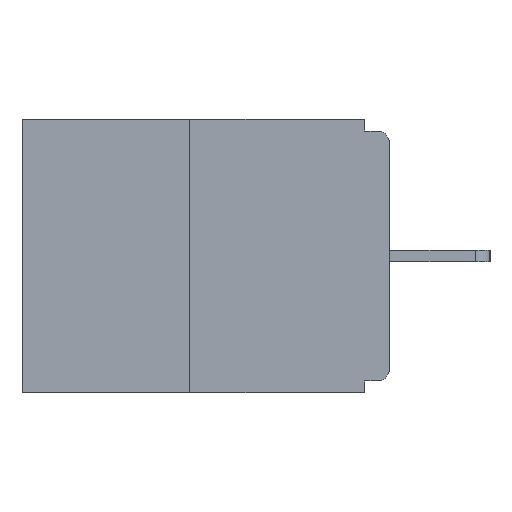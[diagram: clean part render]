
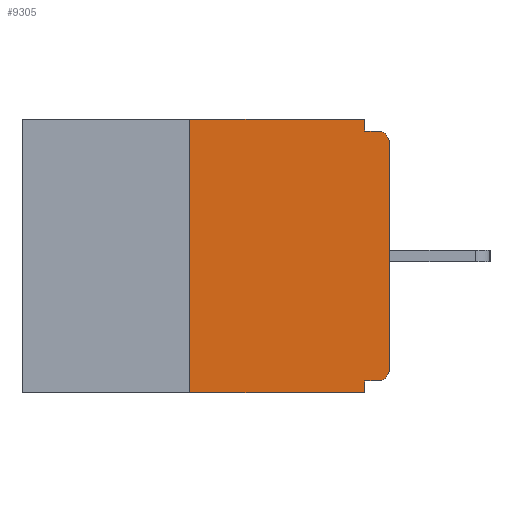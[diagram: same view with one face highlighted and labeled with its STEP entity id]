
A CAD part, left-side view. The second image highlights one B-rep face of the part: STEP entity #9305.
In plain terms, the highlighted planar face has unit normal (-1, 0, 0).
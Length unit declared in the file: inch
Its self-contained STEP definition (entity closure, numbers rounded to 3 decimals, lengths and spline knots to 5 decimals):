
#163 = DIRECTION ( 'NONE',  ( 0., -1., 0. ) ) ;
#285 = VERTEX_POINT ( 'NONE', #2103 ) ;
#522 = EDGE_CURVE ( 'NONE', #285, #22776, #17040, .T. ) ;
#612 = DIRECTION ( 'NONE',  ( 0., 0., -1. ) ) ;
#1006 = CARTESIAN_POINT ( 'NONE',  ( 0., 0.25, 0. ) ) ;
#1192 = LINE ( 'NONE', #10420, #7097 ) ;
#1341 = DIRECTION ( 'NONE',  ( 0., 1., 0. ) ) ;
#1607 = VERTEX_POINT ( 'NONE', #23105 ) ;
#1938 = DIRECTION ( 'NONE',  ( -1., 0., 0. ) ) ;
#2103 = CARTESIAN_POINT ( 'NONE',  ( 0., 0.25, -0.343 ) ) ;
#2117 = ORIENTED_EDGE ( 'NONE', *, *, #6158, .F. ) ;
#3334 = VECTOR ( 'NONE', #4882, 39.37008 ) ;
#4086 = CARTESIAN_POINT ( 'NONE',  ( 0., 0.46, 0. ) ) ;
#4260 = CARTESIAN_POINT ( 'NONE',  ( 0., 0.031, -0.328 ) ) ;
#4323 = DIRECTION ( 'NONE',  ( -1., 0., 0. ) ) ;
#4334 = PLANE ( 'NONE',  #9970 ) ;
#4555 = VERTEX_POINT ( 'NONE', #4260 ) ;
#4598 = AXIS2_PLACEMENT_3D ( 'NONE', #17822, #4323, #9831 ) ;
#4882 = DIRECTION ( 'NONE',  ( 0., 0., -1. ) ) ;
#5003 = LINE ( 'NONE', #12257, #3334 ) ;
#5494 = VERTEX_POINT ( 'NONE', #14697 ) ;
#5523 = ORIENTED_EDGE ( 'NONE', *, *, #24624, .T. ) ;
#5715 = ORIENTED_EDGE ( 'NONE', *, *, #16537, .T. ) ;
#6006 = CARTESIAN_POINT ( 'NONE',  ( 0., 0., -0.03 ) ) ;
#6082 = DIRECTION ( 'NONE',  ( 1., 0., 0. ) ) ;
#6158 = EDGE_CURVE ( 'NONE', #17249, #1607, #17245, .T. ) ;
#6559 = ORIENTED_EDGE ( 'NONE', *, *, #17061, .F. ) ;
#6820 = LINE ( 'NONE', #8567, #7460 ) ;
#7097 = VECTOR ( 'NONE', #8794, 39.37008 ) ;
#7415 = EDGE_CURVE ( 'NONE', #22776, #17249, #22381, .T. ) ;
#7460 = VECTOR ( 'NONE', #1341, 39.37008 ) ;
#7556 = CARTESIAN_POINT ( 'NONE',  ( 0., 0.015, -0.03 ) ) ;
#7636 = ORIENTED_EDGE ( 'NONE', *, *, #7415, .F. ) ;
#8252 = EDGE_CURVE ( 'NONE', #1607, #5494, #13034, .T. ) ;
#8452 = VERTEX_POINT ( 'NONE', #11905 ) ;
#8567 = CARTESIAN_POINT ( 'NONE',  ( 0., 0., -0.328 ) ) ;
#8794 = DIRECTION ( 'NONE',  ( 0., -1., 0. ) ) ;
#8797 = CARTESIAN_POINT ( 'NONE',  ( 0., 0., -0.313 ) ) ;
#9305 = ADVANCED_FACE ( 'NONE', ( #10086 ), #4334, .F. ) ;
#9831 = DIRECTION ( 'NONE',  ( 0., 0., -1. ) ) ;
#9891 = DIRECTION ( 'NONE',  ( 0., 0., -1. ) ) ;
#9970 = AXIS2_PLACEMENT_3D ( 'NONE', #4086, #6082, #612 ) ;
#10086 = FACE_OUTER_BOUND ( 'NONE', #13972, .T. ) ;
#10420 = CARTESIAN_POINT ( 'NONE',  ( 0., 0.46, -0.343 ) ) ;
#11234 = ORIENTED_EDGE ( 'NONE', *, *, #16095, .F. ) ;
#11454 = DIRECTION ( 'NONE',  ( 0., 0., 1. ) ) ;
#11485 = ORIENTED_EDGE ( 'NONE', *, *, #522, .F. ) ;
#11905 = CARTESIAN_POINT ( 'NONE',  ( 0., 0.015, -0.328 ) ) ;
#11989 = CARTESIAN_POINT ( 'NONE',  ( 0., 0.031, -0.343 ) ) ;
#12257 = CARTESIAN_POINT ( 'NONE',  ( 0., 0.031, -0.343 ) ) ;
#12744 = ORIENTED_EDGE ( 'NONE', *, *, #19998, .T. ) ;
#13034 = LINE ( 'NONE', #17250, #19500 ) ;
#13067 = DIRECTION ( 'NONE',  ( 0., 0., 1. ) ) ;
#13758 = CARTESIAN_POINT ( 'NONE',  ( 0., 0.031, 0. ) ) ;
#13887 = ORIENTED_EDGE ( 'NONE', *, *, #8252, .F. ) ;
#13972 = EDGE_LOOP ( 'NONE', ( #7636, #11485, #5715, #6559, #11234, #21787, #12744, #5523, #13887, #2117 ) ) ;
#14697 = CARTESIAN_POINT ( 'NONE',  ( 0., 0.015, -0.015 ) ) ;
#15060 = CARTESIAN_POINT ( 'NONE',  ( 0., 0., 0. ) ) ;
#15184 = LINE ( 'NONE', #15060, #22370 ) ;
#15350 = CIRCLE ( 'NONE', #4598, 0.015 ) ;
#16095 = EDGE_CURVE ( 'NONE', #8452, #4555, #6820, .T. ) ;
#16537 = EDGE_CURVE ( 'NONE', #285, #24034, #1192, .T. ) ;
#16689 = CARTESIAN_POINT ( 'NONE',  ( 0., 0.25, 0. ) ) ;
#17040 = LINE ( 'NONE', #16689, #21193 ) ;
#17061 = EDGE_CURVE ( 'NONE', #4555, #24034, #5003, .T. ) ;
#17245 = LINE ( 'NONE', #13758, #23815 ) ;
#17249 = VERTEX_POINT ( 'NONE', #21214 ) ;
#17250 = CARTESIAN_POINT ( 'NONE',  ( 0., 0., -0.015 ) ) ;
#17822 = CARTESIAN_POINT ( 'NONE',  ( 0., 0.015, -0.313 ) ) ;
#17848 = VERTEX_POINT ( 'NONE', #8797 ) ;
#18068 = VERTEX_POINT ( 'NONE', #6006 ) ;
#18282 = VECTOR ( 'NONE', #20985, 39.37008 ) ;
#19500 = VECTOR ( 'NONE', #163, 39.37008 ) ;
#19998 = EDGE_CURVE ( 'NONE', #17848, #18068, #15184, .T. ) ;
#20985 = DIRECTION ( 'NONE',  ( 0., -1., 0. ) ) ;
#21193 = VECTOR ( 'NONE', #13067, 39.37008 ) ;
#21214 = CARTESIAN_POINT ( 'NONE',  ( 0., 0.031, 0. ) ) ;
#21292 = AXIS2_PLACEMENT_3D ( 'NONE', #7556, #1938, #24303 ) ;
#21787 = ORIENTED_EDGE ( 'NONE', *, *, #24415, .T. ) ;
#22370 = VECTOR ( 'NONE', #11454, 39.37008 ) ;
#22381 = LINE ( 'NONE', #22613, #18282 ) ;
#22613 = CARTESIAN_POINT ( 'NONE',  ( 0., 0.46, 0. ) ) ;
#22776 = VERTEX_POINT ( 'NONE', #1006 ) ;
#23105 = CARTESIAN_POINT ( 'NONE',  ( 0., 0.031, -0.015 ) ) ;
#23815 = VECTOR ( 'NONE', #9891, 39.37008 ) ;
#24034 = VERTEX_POINT ( 'NONE', #11989 ) ;
#24303 = DIRECTION ( 'NONE',  ( 0., 0., -1. ) ) ;
#24415 = EDGE_CURVE ( 'NONE', #8452, #17848, #15350, .T. ) ;
#24479 = CIRCLE ( 'NONE', #21292, 0.015 ) ;
#24624 = EDGE_CURVE ( 'NONE', #18068, #5494, #24479, .T. ) ;
